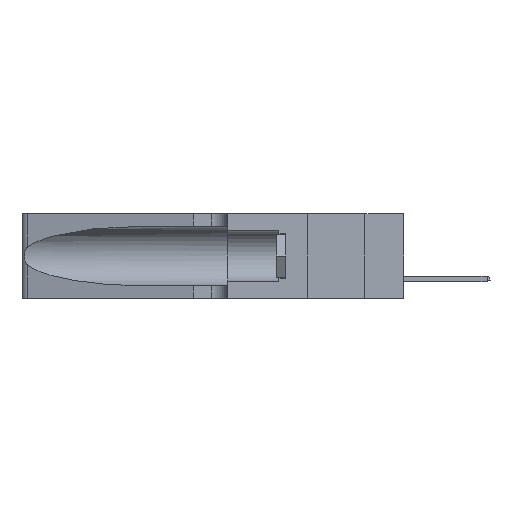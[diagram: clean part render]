
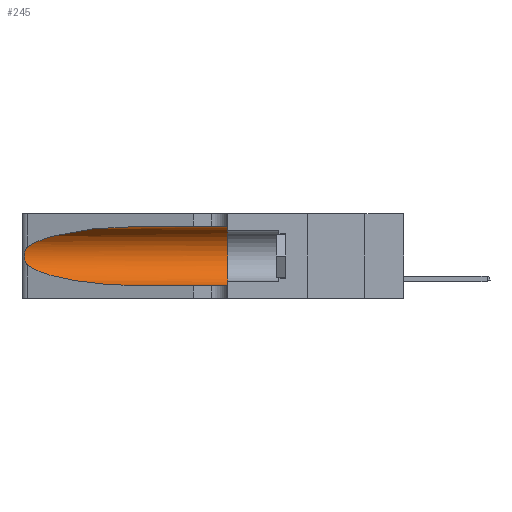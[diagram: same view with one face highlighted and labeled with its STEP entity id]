
A CAD part, left-side view. The second image highlights one B-rep face of the part: STEP entity #245.
In plain terms, the highlighted cylindrical face has radius 3.308 mm (diameter 6.617 mm), a partial arc.
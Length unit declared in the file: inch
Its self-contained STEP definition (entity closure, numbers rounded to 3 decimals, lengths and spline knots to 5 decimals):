
#121 = CARTESIAN_POINT ( 'NONE',  ( 0.25487, 1.22718, 0.22369 ) ) ;
#245 = ADVANCED_FACE ( 'NONE', ( #13064 ), #7913, .F. ) ;
#597 = DIRECTION ( 'NONE',  ( 0., -1., 0. ) ) ;
#2043 = CARTESIAN_POINT ( 'NONE',  ( 0.2373, 1.15595, 0.28018 ) ) ;
#2616 = EDGE_CURVE ( 'NONE', #6856, #12785, #7798, .T. ) ;
#2763 = CARTESIAN_POINT ( 'NONE',  ( 0.25787, 1.23484, 0.2124 ) ) ;
#3233 = CARTESIAN_POINT ( 'NONE',  ( 0.25789, 1.23486, 0.15765 ) ) ;
#3478 = ORIENTED_EDGE ( 'NONE', *, *, #6047, .T. ) ;
#3619 = CARTESIAN_POINT ( 'NONE',  ( 0.25487, 1.22718, 0.22369 ) ) ;
#3889 = DIRECTION ( 'NONE',  ( 0., 1., 0. ) ) ;
#3992 = CARTESIAN_POINT ( 'NONE',  ( 0.1305, 0.35, 0.31525 ) ) ;
#5246 = AXIS2_PLACEMENT_3D ( 'NONE', #10299, #3889, #27897 ) ;
#5550 = CARTESIAN_POINT ( 'NONE',  ( 0.26075, 1.23896, 0.178 ) ) ;
#5981 = DIRECTION ( 'NONE',  ( 0., -1., 0. ) ) ;
#6047 = EDGE_CURVE ( 'NONE', #12785, #7549, #21288, .T. ) ;
#6068 = VERTEX_POINT ( 'NONE', #3992 ) ;
#6078 = CARTESIAN_POINT ( 'NONE',  ( 0.1305, 1.61858, 0.05475 ) ) ;
#6757 = DIRECTION ( 'NONE',  ( 0., 0., -1. ) ) ;
#6856 = VERTEX_POINT ( 'NONE', #3619 ) ;
#7076 = CARTESIAN_POINT ( 'NONE',  ( 0.25555, 1.22994, 0.2215 ) ) ;
#7168 = CARTESIAN_POINT ( 'NONE',  ( 0.26018, 1.23835, 0.19895 ) ) ;
#7363 = CARTESIAN_POINT ( 'NONE',  ( 0.26017, 1.23833, 0.17102 ) ) ;
#7549 = VERTEX_POINT ( 'NONE', #12102 ) ;
#7798 = B_SPLINE_CURVE_WITH_KNOTS ( 'NONE', 3,
 ( #22351, #7076, #24561, #2763, #17915, #7168, #14239, #5550, #7363, #16356, #3233, #9645, #9462, #27165 ),
 .UNSPECIFIED., .F., .F.,
 ( 4, 2, 2, 2, 2, 2, 4 ),
 ( 0., 0.00027, 0.00053, 0.00107, 0.0016, 0.00187, 0.00214 ),
 .UNSPECIFIED. ) ;
#7913 = CYLINDRICAL_SURFACE ( 'NONE', #8765, 0.13025 ) ;
#8149 = ORIENTED_EDGE ( 'NONE', *, *, #27302, .T. ) ;
#8284 = CIRCLE ( 'NONE', #5246, 0.13025 ) ;
#8765 = AXIS2_PLACEMENT_3D ( 'NONE', #9418, #597, #6757 ) ;
#9418 = CARTESIAN_POINT ( 'NONE',  ( 0.1305, 1.61858, 0.185 ) ) ;
#9462 = CARTESIAN_POINT ( 'NONE',  ( 0.25555, 1.22993, 0.14849 ) ) ;
#9645 = CARTESIAN_POINT ( 'NONE',  ( 0.25639, 1.23186, 0.15144 ) ) ;
#10130 = CARTESIAN_POINT ( 'NONE',  ( 0.1305, 0.35, 0.05475 ) ) ;
#10299 = CARTESIAN_POINT ( 'NONE',  ( 0.1305, 0.35, 0.185 ) ) ;
#10529 = ORIENTED_EDGE ( 'NONE', *, *, #2616, .T. ) ;
#10572 = LINE ( 'NONE', #6078, #15713 ) ;
#10749 = EDGE_CURVE ( 'NONE', #16824, #6068, #24113, .T. ) ;
#10759 = CARTESIAN_POINT ( 'NONE',  ( 0.1305, 0.72297, 0.31525 ) ) ;
#10953 = CARTESIAN_POINT ( 'NONE',  ( 0.18966, 0.96281, 0.31525 ) ) ;
#11704 = EDGE_LOOP ( 'NONE', ( #8149, #10529, #3478, #16482, #26845, #18284 ) ) ;
#12102 = CARTESIAN_POINT ( 'NONE',  ( 0.1305, 0.72297, 0.05475 ) ) ;
#12785 = VERTEX_POINT ( 'NONE', #14004 ) ;
#13064 = FACE_OUTER_BOUND ( 'NONE', #11704, .T. ) ;
#14004 = CARTESIAN_POINT ( 'NONE',  ( 0.25487, 1.22718, 0.14631 ) ) ;
#14239 = CARTESIAN_POINT ( 'NONE',  ( 0.26075, 1.23896, 0.19203 ) ) ;
#15055 = EDGE_CURVE ( 'NONE', #6068, #22542, #8284, .T. ) ;
#15126 = CARTESIAN_POINT ( 'NONE',  ( 0.2373, 1.15595, 0.08982 ) ) ;
#15713 = VECTOR ( 'NONE', #5981, 39.37008 ) ;
#16356 = CARTESIAN_POINT ( 'NONE',  ( 0.25856, 1.23593, 0.16098 ) ) ;
#16482 = ORIENTED_EDGE ( 'NONE', *, *, #21331, .T. ) ;
#16824 = VERTEX_POINT ( 'NONE', #20719 ) ;
#17032 = CARTESIAN_POINT ( 'NONE',  ( 0.25487, 1.22718, 0.14631 ) ) ;
#17915 = CARTESIAN_POINT ( 'NONE',  ( 0.25854, 1.2359, 0.20912 ) ) ;
#18284 = ORIENTED_EDGE ( 'NONE', *, *, #10749, .F. ) ;
#20719 = CARTESIAN_POINT ( 'NONE',  ( 0.1305, 0.72297, 0.31525 ) ) ;
#21288 =( BOUNDED_CURVE ( )  B_SPLINE_CURVE ( 3, ( #17032, #15126, #21476, #23793 ),
 .UNSPECIFIED., .F., .F. ) 
 B_SPLINE_CURVE_WITH_KNOTS ( ( 4, 4 ),
 ( 3.44316, 4.71239 ),
 .UNSPECIFIED. ) 
 CURVE ( )  GEOMETRIC_REPRESENTATION_ITEM ( )  RATIONAL_B_SPLINE_CURVE ( ( 1., 0.87, 0.87, 1. ) ) 
 REPRESENTATION_ITEM ( '' )  );
#21331 = EDGE_CURVE ( 'NONE', #7549, #22542, #10572, .T. ) ;
#21476 = CARTESIAN_POINT ( 'NONE',  ( 0.18966, 0.96281, 0.05475 ) ) ;
#22351 = CARTESIAN_POINT ( 'NONE',  ( 0.25487, 1.22718, 0.22369 ) ) ;
#22542 = VERTEX_POINT ( 'NONE', #10130 ) ;
#23793 = CARTESIAN_POINT ( 'NONE',  ( 0.1305, 0.72297, 0.05475 ) ) ;
#24113 = LINE ( 'NONE', #27500, #24789 ) ;
#24561 = CARTESIAN_POINT ( 'NONE',  ( 0.25639, 1.23184, 0.21858 ) ) ;
#24789 = VECTOR ( 'NONE', #25102, 39.37008 ) ;
#25102 = DIRECTION ( 'NONE',  ( 0., -1., 0. ) ) ;
#26845 = ORIENTED_EDGE ( 'NONE', *, *, #15055, .F. ) ;
#27165 = CARTESIAN_POINT ( 'NONE',  ( 0.25487, 1.22718, 0.14631 ) ) ;
#27274 =( BOUNDED_CURVE ( )  B_SPLINE_CURVE ( 3, ( #10759, #10953, #2043, #121 ),
 .UNSPECIFIED., .F., .F. ) 
 B_SPLINE_CURVE_WITH_KNOTS ( ( 4, 4 ),
 ( 1.5708, 2.84003 ),
 .UNSPECIFIED. ) 
 CURVE ( )  GEOMETRIC_REPRESENTATION_ITEM ( )  RATIONAL_B_SPLINE_CURVE ( ( 1., 0.87, 0.87, 1. ) ) 
 REPRESENTATION_ITEM ( '' )  );
#27302 = EDGE_CURVE ( 'NONE', #16824, #6856, #27274, .T. ) ;
#27500 = CARTESIAN_POINT ( 'NONE',  ( 0.1305, 1.61858, 0.31525 ) ) ;
#27897 = DIRECTION ( 'NONE',  ( 0., 0., 1. ) ) ;
